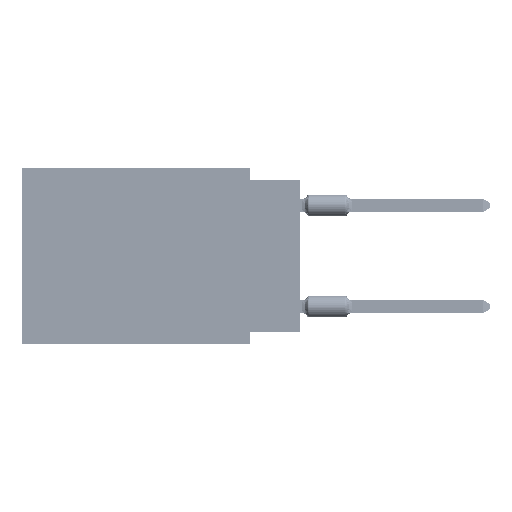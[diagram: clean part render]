
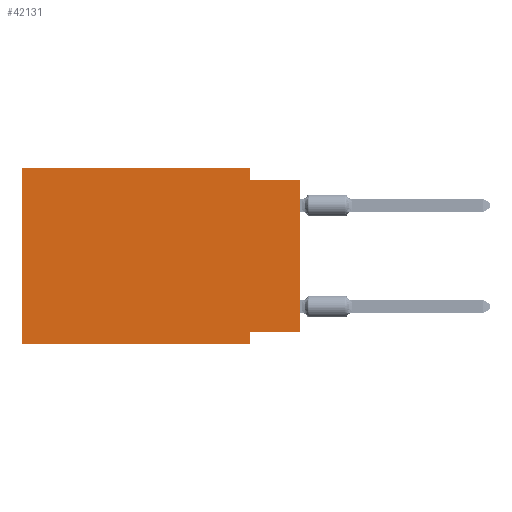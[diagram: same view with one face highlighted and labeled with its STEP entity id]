
A CAD part, left-side view. The second image highlights one B-rep face of the part: STEP entity #42131.
In plain terms, the highlighted planar face has unit normal (-1, 0, 0).
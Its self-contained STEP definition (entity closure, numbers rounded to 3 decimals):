
#664 = DIRECTION ( 'NONE',  ( 0., 0., -1. ) ) ;
#972 = EDGE_CURVE ( 'NONE', #96040, #7722, #74031, .T. ) ;
#1604 = VERTEX_POINT ( 'NONE', #19869 ) ;
#5931 = CARTESIAN_POINT ( 'NONE',  ( 0., 2.54, -8.89 ) ) ;
#7722 = VERTEX_POINT ( 'NONE', #16720 ) ;
#8405 = VECTOR ( 'NONE', #41418, 1000. ) ;
#10428 = CARTESIAN_POINT ( 'NONE',  ( 0., 0., -0.635 ) ) ;
#10536 = LINE ( 'NONE', #33088, #70130 ) ;
#11369 = VERTEX_POINT ( 'NONE', #80445 ) ;
#11526 = CARTESIAN_POINT ( 'NONE',  ( 0., 0., 0. ) ) ;
#13262 = ORIENTED_EDGE ( 'NONE', *, *, #95354, .F. ) ;
#15678 = CARTESIAN_POINT ( 'NONE',  ( 0., 13.97, -8.89 ) ) ;
#16720 = CARTESIAN_POINT ( 'NONE',  ( 0., 2.54, -8.255 ) ) ;
#17171 = EDGE_CURVE ( 'NONE', #18664, #60541, #26986, .T. ) ;
#17373 = CARTESIAN_POINT ( 'NONE',  ( 0., 0., -0.635 ) ) ;
#18664 = VERTEX_POINT ( 'NONE', #15678 ) ;
#19849 = ORIENTED_EDGE ( 'NONE', *, *, #88928, .F. ) ;
#19869 = CARTESIAN_POINT ( 'NONE',  ( 0., 13.97, 0. ) ) ;
#19943 = ORIENTED_EDGE ( 'NONE', *, *, #83909, .T. ) ;
#25555 = ORIENTED_EDGE ( 'NONE', *, *, #41927, .F. ) ;
#26171 = DIRECTION ( 'NONE',  ( 0., 0., -1. ) ) ;
#26986 = LINE ( 'NONE', #87328, #93484 ) ;
#28397 = FACE_OUTER_BOUND ( 'NONE', #87172, .T. ) ;
#28989 = VECTOR ( 'NONE', #664, 1000. ) ;
#30563 = ORIENTED_EDGE ( 'NONE', *, *, #41344, .F. ) ;
#32491 = LINE ( 'NONE', #10428, #58766 ) ;
#33088 = CARTESIAN_POINT ( 'NONE',  ( 0., 13.97, 0. ) ) ;
#34895 = CARTESIAN_POINT ( 'NONE',  ( 0., 13.97, 0. ) ) ;
#35262 = VECTOR ( 'NONE', #52029, 1000. ) ;
#35362 = VERTEX_POINT ( 'NONE', #17373 ) ;
#36243 = DIRECTION ( 'NONE',  ( 0., 0., -1. ) ) ;
#36953 = CARTESIAN_POINT ( 'NONE',  ( 0., 2.54, 0. ) ) ;
#39232 = ORIENTED_EDGE ( 'NONE', *, *, #17171, .T. ) ;
#41344 = EDGE_CURVE ( 'NONE', #7722, #60541, #72287, .T. ) ;
#41418 = DIRECTION ( 'NONE',  ( 0., 0., 1. ) ) ;
#41524 = CARTESIAN_POINT ( 'NONE',  ( 0., 0., -8.255 ) ) ;
#41823 = EDGE_CURVE ( 'NONE', #11369, #46027, #88494, .T. ) ;
#41862 = CARTESIAN_POINT ( 'NONE',  ( 0., 2.54, -8.89 ) ) ;
#41927 = EDGE_CURVE ( 'NONE', #46027, #35362, #32491, .T. ) ;
#42131 = ADVANCED_FACE ( 'NONE', ( #28397 ), #73533, .F. ) ;
#45044 = ORIENTED_EDGE ( 'NONE', *, *, #972, .F. ) ;
#46027 = VERTEX_POINT ( 'NONE', #73331 ) ;
#46043 = CARTESIAN_POINT ( 'NONE',  ( 0., 0., -8.255 ) ) ;
#52029 = DIRECTION ( 'NONE',  ( 0., -1., 0. ) ) ;
#52430 = DIRECTION ( 'NONE',  ( 0., 1., 0. ) ) ;
#58434 = LINE ( 'NONE', #34895, #35262 ) ;
#58766 = VECTOR ( 'NONE', #90412, 1000. ) ;
#60541 = VERTEX_POINT ( 'NONE', #5931 ) ;
#63364 = VECTOR ( 'NONE', #26171, 1000. ) ;
#66946 = ORIENTED_EDGE ( 'NONE', *, *, #41823, .F. ) ;
#69758 = AXIS2_PLACEMENT_3D ( 'NONE', #94650, #87295, #36243 ) ;
#70130 = VECTOR ( 'NONE', #93908, 1000. ) ;
#72287 = LINE ( 'NONE', #41862, #63364 ) ;
#73331 = CARTESIAN_POINT ( 'NONE',  ( 0., 2.54, -0.635 ) ) ;
#73533 = PLANE ( 'NONE',  #69758 ) ;
#74031 = LINE ( 'NONE', #46043, #80563 ) ;
#78715 = LINE ( 'NONE', #11526, #8405 ) ;
#80445 = CARTESIAN_POINT ( 'NONE',  ( 0., 2.54, 0. ) ) ;
#80563 = VECTOR ( 'NONE', #52430, 1000. ) ;
#83909 = EDGE_CURVE ( 'NONE', #96040, #35362, #78715, .T. ) ;
#87172 = EDGE_LOOP ( 'NONE', ( #19943, #25555, #66946, #13262, #19849, #39232, #30563, #45044 ) ) ;
#87295 = DIRECTION ( 'NONE',  ( 1., 0., 0. ) ) ;
#87328 = CARTESIAN_POINT ( 'NONE',  ( 0., 13.97, -8.89 ) ) ;
#88494 = LINE ( 'NONE', #36953, #28989 ) ;
#88928 = EDGE_CURVE ( 'NONE', #18664, #1604, #10536, .T. ) ;
#90412 = DIRECTION ( 'NONE',  ( 0., -1., 0. ) ) ;
#93484 = VECTOR ( 'NONE', #94687, 1000. ) ;
#93908 = DIRECTION ( 'NONE',  ( 0., 0., 1. ) ) ;
#94650 = CARTESIAN_POINT ( 'NONE',  ( 0., 13.97, 0. ) ) ;
#94687 = DIRECTION ( 'NONE',  ( 0., -1., 0. ) ) ;
#95354 = EDGE_CURVE ( 'NONE', #1604, #11369, #58434, .T. ) ;
#96040 = VERTEX_POINT ( 'NONE', #41524 ) ;
